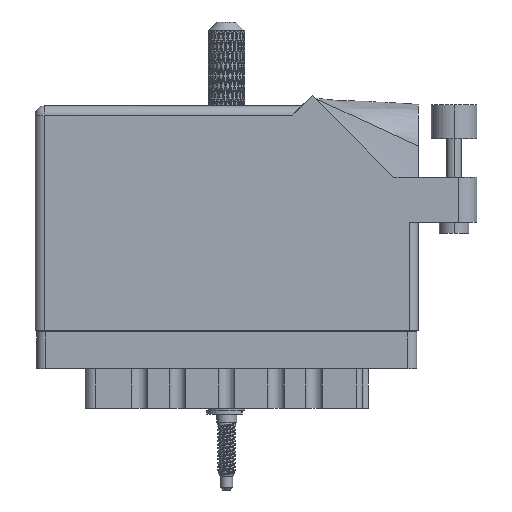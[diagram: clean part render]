
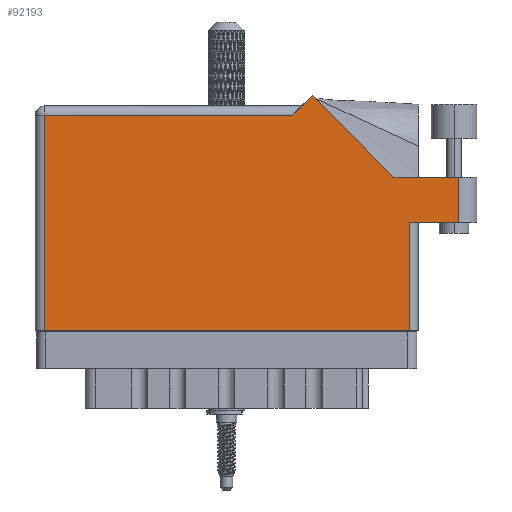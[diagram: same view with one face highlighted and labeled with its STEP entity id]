
A CAD part, front view. The second image highlights one B-rep face of the part: STEP entity #92193.
In plain terms, the highlighted face is planar.
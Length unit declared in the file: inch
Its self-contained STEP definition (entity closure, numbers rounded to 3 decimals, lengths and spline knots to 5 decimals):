
#1271 = DIRECTION ( 'NONE',  ( 0., 1., 0. ) ) ;
#5934 = LINE ( 'NONE', #57501, #109663 ) ;
#16824 = AXIS2_PLACEMENT_3D ( 'NONE', #61467, #70313, #117910 ) ;
#17861 = LINE ( 'NONE', #96108, #88452 ) ;
#20658 = VERTEX_POINT ( 'NONE', #63125 ) ;
#24784 = CARTESIAN_POINT ( 'NONE',  ( 2.44642, 1.044, 0. ) ) ;
#24985 = LINE ( 'NONE', #92531, #55310 ) ;
#25454 = CARTESIAN_POINT ( 'NONE',  ( 2.55, 0., 0. ) ) ;
#28505 = VERTEX_POINT ( 'NONE', #96581 ) ;
#28581 = LINE ( 'NONE', #24784, #104915 ) ;
#30163 = EDGE_CURVE ( 'NONE', #52761, #20658, #64602, .T. ) ;
#30399 = ORIENTED_EDGE ( 'NONE', *, *, #55148, .T. ) ;
#30447 = VECTOR ( 'NONE', #1271, 39.37008 ) ;
#32398 = FACE_OUTER_BOUND ( 'NONE', #91187, .T. ) ;
#33094 = CARTESIAN_POINT ( 'NONE',  ( 1.88971, 1.60071, 0. ) ) ;
#33145 = CARTESIAN_POINT ( 'NONE',  ( 1.757, 1.468, 0. ) ) ;
#34214 = VERTEX_POINT ( 'NONE', #25454 ) ;
#34574 = ORIENTED_EDGE ( 'NONE', *, *, #43693, .T. ) ;
#34824 = ORIENTED_EDGE ( 'NONE', *, *, #41815, .T. ) ;
#35097 = CARTESIAN_POINT ( 'NONE',  ( 0.062, 1.468, 0. ) ) ;
#38594 = DIRECTION ( 'NONE',  ( -1., 0., 0. ) ) ;
#39656 = ORIENTED_EDGE ( 'NONE', *, *, #58913, .T. ) ;
#41815 = EDGE_CURVE ( 'NONE', #46725, #95673, #24985, .T. ) ;
#42360 = VECTOR ( 'NONE', #60496, 39.37008 ) ;
#43162 = CARTESIAN_POINT ( 'NONE',  ( 2.55, 0.737, 0. ) ) ;
#43212 = VECTOR ( 'NONE', #57039, 39.37008 ) ;
#43693 = EDGE_CURVE ( 'NONE', #34214, #64520, #62033, .T. ) ;
#46725 = VERTEX_POINT ( 'NONE', #33145 ) ;
#49406 = DIRECTION ( 'NONE',  ( 1., 0., 0. ) ) ;
#52193 = CARTESIAN_POINT ( 'NONE',  ( 0., 0., 0. ) ) ;
#52761 = VERTEX_POINT ( 'NONE', #54019 ) ;
#52986 = CARTESIAN_POINT ( 'NONE',  ( 3.012, 1.044, 0. ) ) ;
#54019 = CARTESIAN_POINT ( 'NONE',  ( 2.887, 1.044, 0. ) ) ;
#54764 = LINE ( 'NONE', #52193, #73397 ) ;
#54851 = LINE ( 'NONE', #102089, #43212 ) ;
#55148 = EDGE_CURVE ( 'NONE', #103667, #46725, #17861, .T. ) ;
#55310 = VECTOR ( 'NONE', #38594, 39.37008 ) ;
#55931 = EDGE_CURVE ( 'NONE', #85028, #52761, #72658, .T. ) ;
#57039 = DIRECTION ( 'NONE',  ( 0., -1., 0. ) ) ;
#57501 = CARTESIAN_POINT ( 'NONE',  ( 2.612, 0.737, 0. ) ) ;
#58322 = DIRECTION ( 'NONE',  ( -0.707, -0.707, 0. ) ) ;
#58913 = EDGE_CURVE ( 'NONE', #64520, #85028, #5934, .T. ) ;
#60496 = DIRECTION ( 'NONE',  ( 0., 1., 0. ) ) ;
#61467 = CARTESIAN_POINT ( 'NONE',  ( 0., 1.53, 0. ) ) ;
#61712 = VECTOR ( 'NONE', #71875, 39.37008 ) ;
#62033 = LINE ( 'NONE', #85345, #30447 ) ;
#63125 = CARTESIAN_POINT ( 'NONE',  ( 2.44642, 1.044, 0. ) ) ;
#64520 = VERTEX_POINT ( 'NONE', #43162 ) ;
#64602 = LINE ( 'NONE', #52986, #61712 ) ;
#70313 = DIRECTION ( 'NONE',  ( 0., 0., -1. ) ) ;
#71555 = PLANE ( 'NONE',  #16824 ) ;
#71875 = DIRECTION ( 'NONE',  ( -1., 0., 0. ) ) ;
#72542 = EDGE_CURVE ( 'NONE', #28505, #34214, #54764, .T. ) ;
#72658 = LINE ( 'NONE', #100408, #42360 ) ;
#73397 = VECTOR ( 'NONE', #79914, 39.37008 ) ;
#79221 = ORIENTED_EDGE ( 'NONE', *, *, #30163, .T. ) ;
#79914 = DIRECTION ( 'NONE',  ( 1., 0., 0. ) ) ;
#84122 = ORIENTED_EDGE ( 'NONE', *, *, #72542, .T. ) ;
#85028 = VERTEX_POINT ( 'NONE', #87578 ) ;
#85168 = ORIENTED_EDGE ( 'NONE', *, *, #112191, .T. ) ;
#85345 = CARTESIAN_POINT ( 'NONE',  ( 2.55, 0.737, 0. ) ) ;
#87578 = CARTESIAN_POINT ( 'NONE',  ( 2.887, 0.737, 0. ) ) ;
#88059 = ORIENTED_EDGE ( 'NONE', *, *, #55931, .T. ) ;
#88452 = VECTOR ( 'NONE', #58322, 39.37008 ) ;
#89986 = DIRECTION ( 'NONE',  ( -0.707, 0.707, 0. ) ) ;
#91187 = EDGE_LOOP ( 'NONE', ( #39656, #88059, #79221, #85168, #30399, #34824, #110118, #84122, #34574 ) ) ;
#92193 = ADVANCED_FACE ( 'NONE', ( #32398 ), #71555, .F. ) ;
#92531 = CARTESIAN_POINT ( 'NONE',  ( 0., 1.468, 0. ) ) ;
#95673 = VERTEX_POINT ( 'NONE', #35097 ) ;
#96108 = CARTESIAN_POINT ( 'NONE',  ( 1.819, 1.53, 0. ) ) ;
#96581 = CARTESIAN_POINT ( 'NONE',  ( 0.062, 0., 0. ) ) ;
#100408 = CARTESIAN_POINT ( 'NONE',  ( 2.887, 1.044, 0. ) ) ;
#102089 = CARTESIAN_POINT ( 'NONE',  ( 0.062, 0., 0. ) ) ;
#103667 = VERTEX_POINT ( 'NONE', #33094 ) ;
#104915 = VECTOR ( 'NONE', #89986, 39.37008 ) ;
#109663 = VECTOR ( 'NONE', #49406, 39.37008 ) ;
#110118 = ORIENTED_EDGE ( 'NONE', *, *, #118936, .T. ) ;
#112191 = EDGE_CURVE ( 'NONE', #20658, #103667, #28581, .T. ) ;
#117910 = DIRECTION ( 'NONE',  ( -1., 0., 0. ) ) ;
#118936 = EDGE_CURVE ( 'NONE', #95673, #28505, #54851, .T. ) ;
